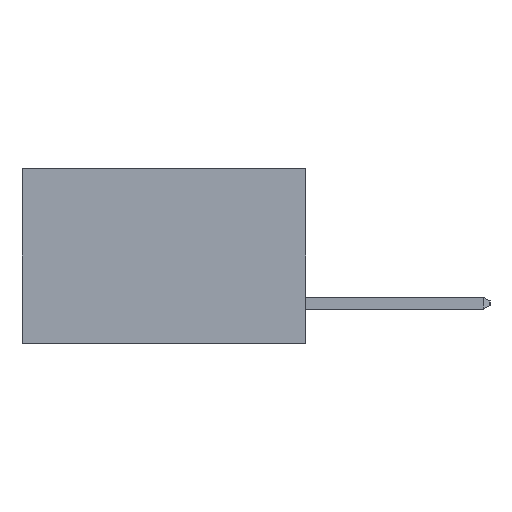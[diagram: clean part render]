
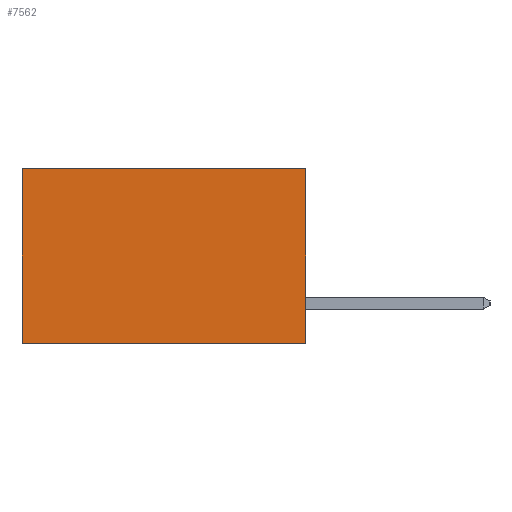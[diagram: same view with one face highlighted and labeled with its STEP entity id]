
A CAD part, left-side view. The second image highlights one B-rep face of the part: STEP entity #7562.
In plain terms, the highlighted planar face has unit normal (-1, 0, 0).
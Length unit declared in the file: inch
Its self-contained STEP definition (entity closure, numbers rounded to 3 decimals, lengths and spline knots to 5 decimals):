
#1226 = LINE ( 'NONE', #20574, #6165 ) ;
#1736 = VERTEX_POINT ( 'NONE', #9897 ) ;
#1875 = LINE ( 'NONE', #2415, #22698 ) ;
#2108 = DIRECTION ( 'NONE',  ( 0., 0., -1. ) ) ;
#2415 = CARTESIAN_POINT ( 'NONE',  ( 0.298, 0., -0.37 ) ) ;
#3372 = EDGE_CURVE ( 'NONE', #8414, #1736, #6784, .T. ) ;
#3986 = ORIENTED_EDGE ( 'NONE', *, *, #15060, .F. ) ;
#4227 = CARTESIAN_POINT ( 'NONE',  ( 0.298, 0.6, 0. ) ) ;
#5125 = VERTEX_POINT ( 'NONE', #5175 ) ;
#5175 = CARTESIAN_POINT ( 'NONE',  ( 0.298, 0.6, -0.37 ) ) ;
#5798 = VECTOR ( 'NONE', #2108, 39.37008 ) ;
#6165 = VECTOR ( 'NONE', #14478, 39.37008 ) ;
#6466 = LINE ( 'NONE', #4227, #5798 ) ;
#6784 = LINE ( 'NONE', #17101, #11674 ) ;
#7422 = PLANE ( 'NONE',  #16027 ) ;
#7562 = ADVANCED_FACE ( 'NONE', ( #10071 ), #7422, .F. ) ;
#7853 = VERTEX_POINT ( 'NONE', #14598 ) ;
#8414 = VERTEX_POINT ( 'NONE', #24371 ) ;
#9270 = ORIENTED_EDGE ( 'NONE', *, *, #22963, .F. ) ;
#9534 = CARTESIAN_POINT ( 'NONE',  ( 0.298, 0., 0. ) ) ;
#9897 = CARTESIAN_POINT ( 'NONE',  ( 0.298, 0.6, 0. ) ) ;
#10071 = FACE_OUTER_BOUND ( 'NONE', #25427, .T. ) ;
#11674 = VECTOR ( 'NONE', #21726, 39.37008 ) ;
#12297 = ORIENTED_EDGE ( 'NONE', *, *, #12582, .T. ) ;
#12582 = EDGE_CURVE ( 'NONE', #1736, #5125, #6466, .T. ) ;
#14272 = ORIENTED_EDGE ( 'NONE', *, *, #3372, .T. ) ;
#14478 = DIRECTION ( 'NONE',  ( 0., 0., -1. ) ) ;
#14598 = CARTESIAN_POINT ( 'NONE',  ( 0.298, 0., -0.37 ) ) ;
#15060 = EDGE_CURVE ( 'NONE', #7853, #5125, #1875, .T. ) ;
#16027 = AXIS2_PLACEMENT_3D ( 'NONE', #9534, #22143, #22246 ) ;
#17101 = CARTESIAN_POINT ( 'NONE',  ( 0.298, 0., 0. ) ) ;
#20574 = CARTESIAN_POINT ( 'NONE',  ( 0.298, 0., 0. ) ) ;
#21134 = DIRECTION ( 'NONE',  ( 0., 1., 0. ) ) ;
#21726 = DIRECTION ( 'NONE',  ( 0., 1., 0. ) ) ;
#22143 = DIRECTION ( 'NONE',  ( 1., 0., 0. ) ) ;
#22246 = DIRECTION ( 'NONE',  ( 0., 0., -1. ) ) ;
#22698 = VECTOR ( 'NONE', #21134, 39.37008 ) ;
#22963 = EDGE_CURVE ( 'NONE', #8414, #7853, #1226, .T. ) ;
#24371 = CARTESIAN_POINT ( 'NONE',  ( 0.298, 0., 0. ) ) ;
#25427 = EDGE_LOOP ( 'NONE', ( #12297, #3986, #9270, #14272 ) ) ;
